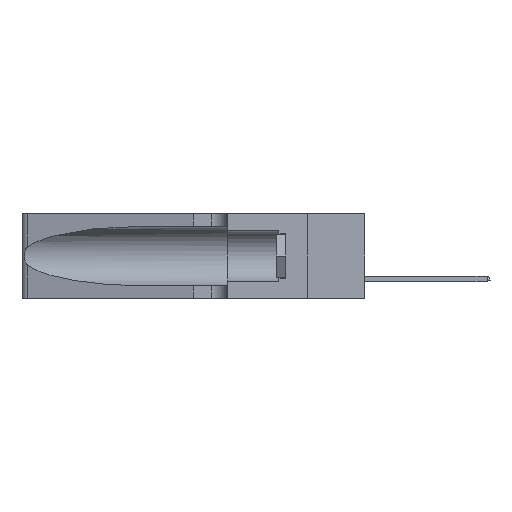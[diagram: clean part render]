
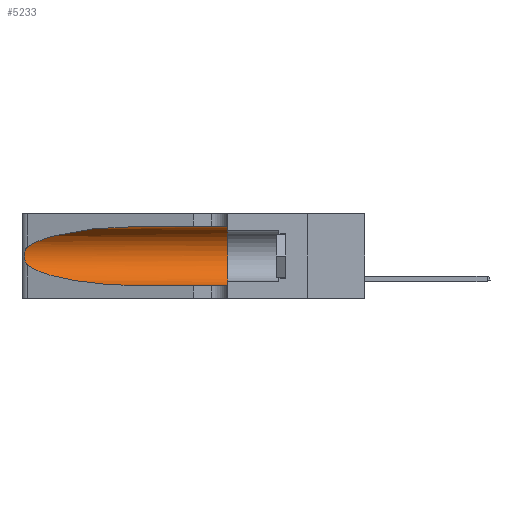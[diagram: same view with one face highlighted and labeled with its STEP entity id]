
A CAD part, left-side view. The second image highlights one B-rep face of the part: STEP entity #5233.
In plain terms, the highlighted cylindrical face has radius 3.308 mm (diameter 6.617 mm), a partial arc.
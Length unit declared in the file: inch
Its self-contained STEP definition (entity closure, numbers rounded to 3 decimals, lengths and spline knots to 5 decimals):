
#354 = CARTESIAN_POINT ( 'NONE',  ( 0.1305, 0.35, 0.05475 ) ) ;
#516 = CARTESIAN_POINT ( 'NONE',  ( 0.2373, 1.15595, 0.28018 ) ) ;
#661 = ORIENTED_EDGE ( 'NONE', *, *, #13539, .T. ) ;
#963 = EDGE_CURVE ( 'NONE', #22565, #5755, #22486, .T. ) ;
#1718 = VERTEX_POINT ( 'NONE', #20439 ) ;
#1939 = EDGE_CURVE ( 'NONE', #1718, #5102, #3255, .T. ) ;
#2262 = CARTESIAN_POINT ( 'NONE',  ( 0.1305, 0.35, 0.31525 ) ) ;
#2740 = CYLINDRICAL_SURFACE ( 'NONE', #6089, 0.13025 ) ;
#3255 = LINE ( 'NONE', #7495, #11936 ) ;
#3787 = DIRECTION ( 'NONE',  ( 0., -1., 0. ) ) ;
#4287 = DIRECTION ( 'NONE',  ( 0., 0., -1. ) ) ;
#5102 = VERTEX_POINT ( 'NONE', #354 ) ;
#5233 = ADVANCED_FACE ( 'NONE', ( #22360 ), #2740, .F. ) ;
#5666 = CARTESIAN_POINT ( 'NONE',  ( 0.25639, 1.23186, 0.15144 ) ) ;
#5755 = VERTEX_POINT ( 'NONE', #17347 ) ;
#6089 = AXIS2_PLACEMENT_3D ( 'NONE', #12620, #3787, #4287 ) ;
#6542 = EDGE_LOOP ( 'NONE', ( #6687, #661, #11137, #6711, #22740, #20474 ) ) ;
#6687 = ORIENTED_EDGE ( 'NONE', *, *, #963, .T. ) ;
#6711 = ORIENTED_EDGE ( 'NONE', *, *, #1939, .T. ) ;
#6724 = CARTESIAN_POINT ( 'NONE',  ( 0.1305, 1.61858, 0.31525 ) ) ;
#7495 = CARTESIAN_POINT ( 'NONE',  ( 0.1305, 1.61858, 0.05475 ) ) ;
#8415 = CIRCLE ( 'NONE', #16551, 0.13025 ) ;
#9032 = EDGE_CURVE ( 'NONE', #22565, #11872, #19625, .T. ) ;
#9034 = CARTESIAN_POINT ( 'NONE',  ( 0.26018, 1.23835, 0.19895 ) ) ;
#9268 = CARTESIAN_POINT ( 'NONE',  ( 0.25555, 1.22993, 0.14849 ) ) ;
#9351 = CARTESIAN_POINT ( 'NONE',  ( 0.25789, 1.23486, 0.15765 ) ) ;
#10202 = DIRECTION ( 'NONE',  ( 0., 1., 0. ) ) ;
#10736 = CARTESIAN_POINT ( 'NONE',  ( 0.25639, 1.23184, 0.21858 ) ) ;
#11137 = ORIENTED_EDGE ( 'NONE', *, *, #16778, .T. ) ;
#11207 = CARTESIAN_POINT ( 'NONE',  ( 0.18966, 0.96281, 0.31525 ) ) ;
#11872 = VERTEX_POINT ( 'NONE', #2262 ) ;
#11936 = VECTOR ( 'NONE', #15480, 39.37008 ) ;
#12506 = CARTESIAN_POINT ( 'NONE',  ( 0.25854, 1.2359, 0.20912 ) ) ;
#12583 = CARTESIAN_POINT ( 'NONE',  ( 0.26075, 1.23896, 0.19203 ) ) ;
#12620 = CARTESIAN_POINT ( 'NONE',  ( 0.1305, 1.61858, 0.185 ) ) ;
#12966 = CARTESIAN_POINT ( 'NONE',  ( 0.25856, 1.23593, 0.16098 ) ) ;
#13539 = EDGE_CURVE ( 'NONE', #5755, #22478, #17035, .T. ) ;
#14577 =( BOUNDED_CURVE ( )  B_SPLINE_CURVE ( 3, ( #18802, #16904, #15151, #18726 ),
 .UNSPECIFIED., .F., .F. ) 
 B_SPLINE_CURVE_WITH_KNOTS ( ( 4, 4 ),
 ( 3.44316, 4.71239 ),
 .UNSPECIFIED. ) 
 CURVE ( )  GEOMETRIC_REPRESENTATION_ITEM ( )  RATIONAL_B_SPLINE_CURVE ( ( 1., 0.87, 0.87, 1. ) ) 
 REPRESENTATION_ITEM ( '' )  );
#14606 = EDGE_CURVE ( 'NONE', #11872, #5102, #8415, .T. ) ;
#14626 = CARTESIAN_POINT ( 'NONE',  ( 0.26017, 1.23833, 0.17102 ) ) ;
#14813 = VECTOR ( 'NONE', #21074, 39.37008 ) ;
#15151 = CARTESIAN_POINT ( 'NONE',  ( 0.18966, 0.96281, 0.05475 ) ) ;
#15480 = DIRECTION ( 'NONE',  ( 0., -1., 0. ) ) ;
#15503 = CARTESIAN_POINT ( 'NONE',  ( 0.1305, 0.35, 0.185 ) ) ;
#15673 = DIRECTION ( 'NONE',  ( 0., 0., 1. ) ) ;
#16093 = CARTESIAN_POINT ( 'NONE',  ( 0.25487, 1.22718, 0.14631 ) ) ;
#16551 = AXIS2_PLACEMENT_3D ( 'NONE', #15503, #10202, #15673 ) ;
#16778 = EDGE_CURVE ( 'NONE', #22478, #1718, #14577, .T. ) ;
#16904 = CARTESIAN_POINT ( 'NONE',  ( 0.2373, 1.15595, 0.08982 ) ) ;
#16925 = CARTESIAN_POINT ( 'NONE',  ( 0.25487, 1.22718, 0.22369 ) ) ;
#17035 = B_SPLINE_CURVE_WITH_KNOTS ( 'NONE', 3,
 ( #19613, #21563, #10736, #23271, #12506, #9034, #12583, #23033, #14626, #12966, #9351, #5666, #9268, #19850 ),
 .UNSPECIFIED., .F., .F.,
 ( 4, 2, 2, 2, 2, 2, 4 ),
 ( 0., 0.00027, 0.00053, 0.00107, 0.0016, 0.00187, 0.00214 ),
 .UNSPECIFIED. ) ;
#17347 = CARTESIAN_POINT ( 'NONE',  ( 0.25487, 1.22718, 0.22369 ) ) ;
#18726 = CARTESIAN_POINT ( 'NONE',  ( 0.1305, 0.72297, 0.05475 ) ) ;
#18802 = CARTESIAN_POINT ( 'NONE',  ( 0.25487, 1.22718, 0.14631 ) ) ;
#19613 = CARTESIAN_POINT ( 'NONE',  ( 0.25487, 1.22718, 0.22369 ) ) ;
#19625 = LINE ( 'NONE', #6724, #14813 ) ;
#19850 = CARTESIAN_POINT ( 'NONE',  ( 0.25487, 1.22718, 0.14631 ) ) ;
#20244 = CARTESIAN_POINT ( 'NONE',  ( 0.1305, 0.72297, 0.31525 ) ) ;
#20439 = CARTESIAN_POINT ( 'NONE',  ( 0.1305, 0.72297, 0.05475 ) ) ;
#20474 = ORIENTED_EDGE ( 'NONE', *, *, #9032, .F. ) ;
#21074 = DIRECTION ( 'NONE',  ( 0., -1., 0. ) ) ;
#21563 = CARTESIAN_POINT ( 'NONE',  ( 0.25555, 1.22994, 0.2215 ) ) ;
#21661 = CARTESIAN_POINT ( 'NONE',  ( 0.1305, 0.72297, 0.31525 ) ) ;
#22360 = FACE_OUTER_BOUND ( 'NONE', #6542, .T. ) ;
#22478 = VERTEX_POINT ( 'NONE', #16093 ) ;
#22486 =( BOUNDED_CURVE ( )  B_SPLINE_CURVE ( 3, ( #20244, #11207, #516, #16925 ),
 .UNSPECIFIED., .F., .F. ) 
 B_SPLINE_CURVE_WITH_KNOTS ( ( 4, 4 ),
 ( 1.5708, 2.84003 ),
 .UNSPECIFIED. ) 
 CURVE ( )  GEOMETRIC_REPRESENTATION_ITEM ( )  RATIONAL_B_SPLINE_CURVE ( ( 1., 0.87, 0.87, 1. ) ) 
 REPRESENTATION_ITEM ( '' )  );
#22565 = VERTEX_POINT ( 'NONE', #21661 ) ;
#22740 = ORIENTED_EDGE ( 'NONE', *, *, #14606, .F. ) ;
#23033 = CARTESIAN_POINT ( 'NONE',  ( 0.26075, 1.23896, 0.178 ) ) ;
#23271 = CARTESIAN_POINT ( 'NONE',  ( 0.25787, 1.23484, 0.2124 ) ) ;
